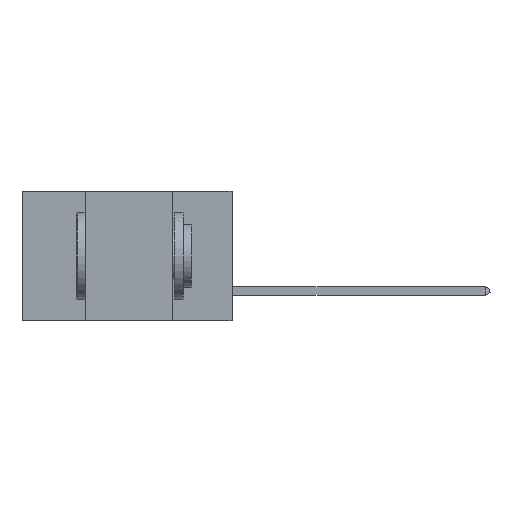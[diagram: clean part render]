
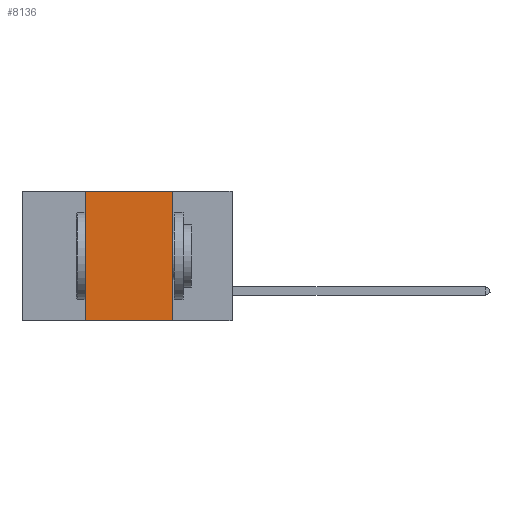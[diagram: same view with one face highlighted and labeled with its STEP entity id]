
A CAD part, left-side view. The second image highlights one B-rep face of the part: STEP entity #8136.
In plain terms, the highlighted planar face has unit normal (-1, 0, 0).
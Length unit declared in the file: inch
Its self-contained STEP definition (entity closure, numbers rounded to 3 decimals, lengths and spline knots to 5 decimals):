
#1 = EDGE_CURVE ( 'NONE', #1358, #10525, #8776, .T. ) ;
#532 = CARTESIAN_POINT ( 'NONE',  ( 0., 0.17, 0. ) ) ;
#755 = VECTOR ( 'NONE', #14215, 39.37008 ) ;
#958 = LINE ( 'NONE', #5537, #755 ) ;
#1358 = VERTEX_POINT ( 'NONE', #14318 ) ;
#1823 = PLANE ( 'NONE',  #13220 ) ;
#3521 = ORIENTED_EDGE ( 'NONE', *, *, #13763, .F. ) ;
#3532 = EDGE_CURVE ( 'NONE', #14929, #4158, #11047, .T. ) ;
#3903 = DIRECTION ( 'NONE',  ( 0., 0., 1. ) ) ;
#4158 = VERTEX_POINT ( 'NONE', #5883 ) ;
#4234 = DIRECTION ( 'NONE',  ( 1., 0., 0. ) ) ;
#5418 = VECTOR ( 'NONE', #3903, 39.37008 ) ;
#5537 = CARTESIAN_POINT ( 'NONE',  ( 0., 0.6, 0. ) ) ;
#5779 = EDGE_CURVE ( 'NONE', #1358, #4158, #10835, .T. ) ;
#5883 = CARTESIAN_POINT ( 'NONE',  ( 0., 0.17, -0.37 ) ) ;
#6129 = VECTOR ( 'NONE', #7503, 39.37008 ) ;
#7457 = ORIENTED_EDGE ( 'NONE', *, *, #3532, .F. ) ;
#7503 = DIRECTION ( 'NONE',  ( 0., -1., 0. ) ) ;
#7531 = CARTESIAN_POINT ( 'NONE',  ( 0., 0.42, 0. ) ) ;
#8136 = ADVANCED_FACE ( 'NONE', ( #10187 ), #1823, .F. ) ;
#8776 = LINE ( 'NONE', #11343, #5418 ) ;
#9298 = DIRECTION ( 'NONE',  ( 0., 0., -1. ) ) ;
#9306 = CARTESIAN_POINT ( 'NONE',  ( 0., 0.6, 0. ) ) ;
#10187 = FACE_OUTER_BOUND ( 'NONE', #15603, .T. ) ;
#10525 = VERTEX_POINT ( 'NONE', #7531 ) ;
#10835 = LINE ( 'NONE', #14876, #6129 ) ;
#11047 = LINE ( 'NONE', #532, #15763 ) ;
#11343 = CARTESIAN_POINT ( 'NONE',  ( 0., 0.42, 0. ) ) ;
#12610 = ORIENTED_EDGE ( 'NONE', *, *, #5779, .T. ) ;
#13000 = DIRECTION ( 'NONE',  ( 0., 0., -1. ) ) ;
#13220 = AXIS2_PLACEMENT_3D ( 'NONE', #9306, #4234, #13000 ) ;
#13763 = EDGE_CURVE ( 'NONE', #10525, #14929, #958, .T. ) ;
#14215 = DIRECTION ( 'NONE',  ( 0., -1., 0. ) ) ;
#14318 = CARTESIAN_POINT ( 'NONE',  ( 0., 0.42, -0.37 ) ) ;
#14876 = CARTESIAN_POINT ( 'NONE',  ( 0., 0.6, -0.37 ) ) ;
#14929 = VERTEX_POINT ( 'NONE', #15766 ) ;
#15603 = EDGE_LOOP ( 'NONE', ( #7457, #3521, #15996, #12610 ) ) ;
#15763 = VECTOR ( 'NONE', #9298, 39.37008 ) ;
#15766 = CARTESIAN_POINT ( 'NONE',  ( 0., 0.17, 0. ) ) ;
#15996 = ORIENTED_EDGE ( 'NONE', *, *, #1, .F. ) ;
